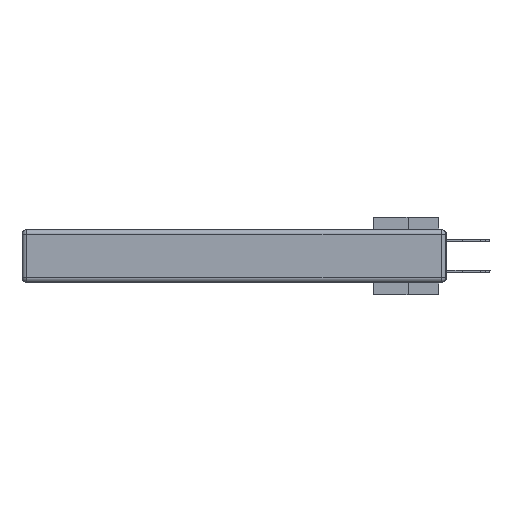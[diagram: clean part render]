
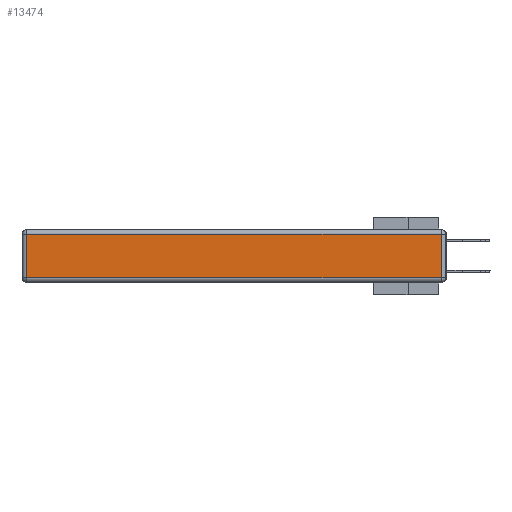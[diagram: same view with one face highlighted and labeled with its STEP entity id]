
A CAD part, left-side view. The second image highlights one B-rep face of the part: STEP entity #13474.
In plain terms, the highlighted planar face has unit normal (-1, 0, 0).
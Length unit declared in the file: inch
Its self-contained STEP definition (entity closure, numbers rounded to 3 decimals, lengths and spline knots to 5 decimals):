
#620 = EDGE_CURVE ( 'NONE', #10329, #12429, #18521, .T. ) ;
#686 = ORIENTED_EDGE ( 'NONE', *, *, #27186, .T. ) ;
#2292 = DIRECTION ( 'NONE',  ( 0., 0., -1. ) ) ;
#3629 = CARTESIAN_POINT ( 'NONE',  ( 0., 2.75, -0.03 ) ) ;
#5755 = EDGE_CURVE ( 'NONE', #12429, #16346, #15355, .T. ) ;
#6000 = CARTESIAN_POINT ( 'NONE',  ( 0., 2.72, -0.313 ) ) ;
#6178 = DIRECTION ( 'NONE',  ( 0., 1., 0. ) ) ;
#7014 = CARTESIAN_POINT ( 'NONE',  ( 0., 2.72, -0.343 ) ) ;
#8423 = VECTOR ( 'NONE', #9248, 39.37008 ) ;
#9248 = DIRECTION ( 'NONE',  ( 0., -1., 0. ) ) ;
#9920 = CARTESIAN_POINT ( 'NONE',  ( 0., 0.03, -0.313 ) ) ;
#10329 = VERTEX_POINT ( 'NONE', #15627 ) ;
#11156 = LINE ( 'NONE', #16138, #29117 ) ;
#11556 = FACE_OUTER_BOUND ( 'NONE', #23394, .T. ) ;
#12429 = VERTEX_POINT ( 'NONE', #6000 ) ;
#13474 = ADVANCED_FACE ( 'NONE', ( #11556 ), #21183, .T. ) ;
#14094 = EDGE_CURVE ( 'NONE', #16346, #23807, #11156, .T. ) ;
#14396 = VECTOR ( 'NONE', #2292, 39.37008 ) ;
#15355 = LINE ( 'NONE', #27524, #8423 ) ;
#15627 = CARTESIAN_POINT ( 'NONE',  ( 0., 2.72, -0.03 ) ) ;
#15796 = DIRECTION ( 'NONE',  ( 0., 0., 1. ) ) ;
#15908 = CARTESIAN_POINT ( 'NONE',  ( 0., 0.03, -0.03 ) ) ;
#15934 = CARTESIAN_POINT ( 'NONE',  ( 0., 0., -0.343 ) ) ;
#16053 = DIRECTION ( 'NONE',  ( -1., 0., 0. ) ) ;
#16138 = CARTESIAN_POINT ( 'NONE',  ( 0., 0.03, -0.343 ) ) ;
#16346 = VERTEX_POINT ( 'NONE', #9920 ) ;
#18521 = LINE ( 'NONE', #7014, #14396 ) ;
#18693 = DIRECTION ( 'NONE',  ( 0., 0., 1. ) ) ;
#20960 = AXIS2_PLACEMENT_3D ( 'NONE', #15934, #16053, #18693 ) ;
#21183 = PLANE ( 'NONE',  #20960 ) ;
#23394 = EDGE_LOOP ( 'NONE', ( #23968, #29424, #686, #32293 ) ) ;
#23629 = VECTOR ( 'NONE', #6178, 39.37008 ) ;
#23807 = VERTEX_POINT ( 'NONE', #15908 ) ;
#23968 = ORIENTED_EDGE ( 'NONE', *, *, #5755, .T. ) ;
#27186 = EDGE_CURVE ( 'NONE', #23807, #10329, #32256, .T. ) ;
#27524 = CARTESIAN_POINT ( 'NONE',  ( 0., 0., -0.313 ) ) ;
#29117 = VECTOR ( 'NONE', #15796, 39.37008 ) ;
#29424 = ORIENTED_EDGE ( 'NONE', *, *, #14094, .T. ) ;
#32256 = LINE ( 'NONE', #3629, #23629 ) ;
#32293 = ORIENTED_EDGE ( 'NONE', *, *, #620, .T. ) ;
